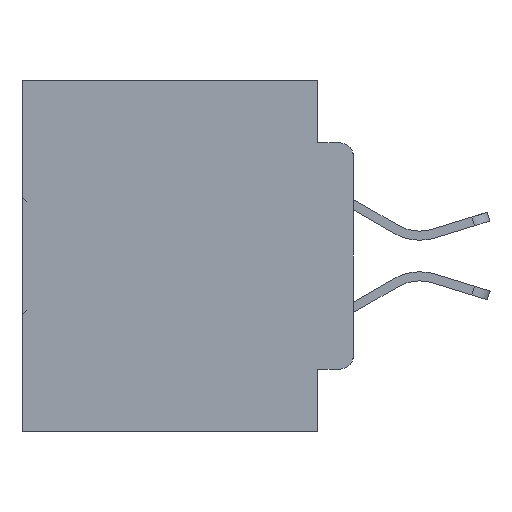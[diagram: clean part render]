
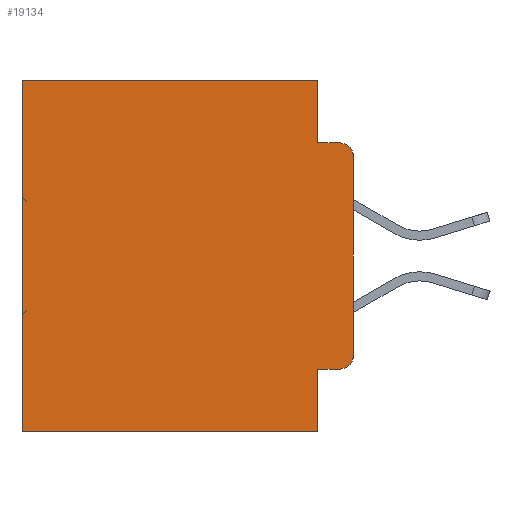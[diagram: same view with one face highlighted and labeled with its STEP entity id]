
A CAD part, left-side view. The second image highlights one B-rep face of the part: STEP entity #19134.
In plain terms, the highlighted planar face has unit normal (-1, 0, 0).
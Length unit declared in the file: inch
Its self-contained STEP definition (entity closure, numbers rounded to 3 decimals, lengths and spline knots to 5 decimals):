
#484 = EDGE_CURVE ( 'NONE', #14846, #5418, #13066, .T. ) ;
#503 = CIRCLE ( 'NONE', #20669, 0.02 ) ;
#848 = PLANE ( 'NONE',  #13218 ) ;
#1187 = LINE ( 'NONE', #32046, #17365 ) ;
#1809 = LINE ( 'NONE', #28675, #14459 ) ;
#2799 = CARTESIAN_POINT ( 'NONE',  ( 0.298, 0.051, 0. ) ) ;
#3646 = VECTOR ( 'NONE', #20056, 39.37008 ) ;
#3702 = VERTEX_POINT ( 'NONE', #13424 ) ;
#3915 = CARTESIAN_POINT ( 'NONE',  ( 0.298, 0., 0. ) ) ;
#3969 = DIRECTION ( 'NONE',  ( 0., -1., 0. ) ) ;
#4075 = EDGE_CURVE ( 'NONE', #13314, #26047, #28355, .T. ) ;
#4445 = ORIENTED_EDGE ( 'NONE', *, *, #15687, .F. ) ;
#4555 = CARTESIAN_POINT ( 'NONE',  ( 0.298, 0.051, -0.5 ) ) ;
#5418 = VERTEX_POINT ( 'NONE', #7967 ) ;
#6611 = VECTOR ( 'NONE', #29232, 39.37008 ) ;
#6970 = EDGE_CURVE ( 'NONE', #30090, #22566, #26677, .T. ) ;
#7066 = DIRECTION ( 'NONE',  ( -1., 0., 0. ) ) ;
#7967 = CARTESIAN_POINT ( 'NONE',  ( 0.298, 0.02, -0.0885 ) ) ;
#8965 = VECTOR ( 'NONE', #35648, 39.37008 ) ;
#8967 = CIRCLE ( 'NONE', #18180, 0.02 ) ;
#9166 = DIRECTION ( 'NONE',  ( 0., 0., -1. ) ) ;
#10667 = LINE ( 'NONE', #12830, #6611 ) ;
#11584 = ORIENTED_EDGE ( 'NONE', *, *, #17065, .F. ) ;
#12199 = DIRECTION ( 'NONE',  ( 0., 0., -1. ) ) ;
#12467 = DIRECTION ( 'NONE',  ( 0., 0., -1. ) ) ;
#12616 = CARTESIAN_POINT ( 'NONE',  ( 0.298, 0., 0. ) ) ;
#12733 = ORIENTED_EDGE ( 'NONE', *, *, #28550, .F. ) ;
#12830 = CARTESIAN_POINT ( 'NONE',  ( 0.298, 0., -0.5 ) ) ;
#13066 = LINE ( 'NONE', #34368, #33563 ) ;
#13218 = AXIS2_PLACEMENT_3D ( 'NONE', #3915, #17276, #9166 ) ;
#13314 = VERTEX_POINT ( 'NONE', #18774 ) ;
#13424 = CARTESIAN_POINT ( 'NONE',  ( 0.298, 0., -0.1085 ) ) ;
#14459 = VECTOR ( 'NONE', #3969, 39.37008 ) ;
#14616 = ORIENTED_EDGE ( 'NONE', *, *, #22593, .T. ) ;
#14752 = FACE_OUTER_BOUND ( 'NONE', #29911, .T. ) ;
#14810 = DIRECTION ( 'NONE',  ( -1., 0., 0. ) ) ;
#14846 = VERTEX_POINT ( 'NONE', #15493 ) ;
#14872 = ORIENTED_EDGE ( 'NONE', *, *, #30583, .T. ) ;
#14900 = CARTESIAN_POINT ( 'NONE',  ( 0.298, 0.473, 0. ) ) ;
#15001 = CARTESIAN_POINT ( 'NONE',  ( 0.298, 0.02, -0.4115 ) ) ;
#15191 = CARTESIAN_POINT ( 'NONE',  ( 0.298, 0.02, -0.1085 ) ) ;
#15493 = CARTESIAN_POINT ( 'NONE',  ( 0.298, 0.051, -0.0885 ) ) ;
#15687 = EDGE_CURVE ( 'NONE', #3702, #35352, #29051, .T. ) ;
#16930 = VERTEX_POINT ( 'NONE', #15001 ) ;
#17065 = EDGE_CURVE ( 'NONE', #26047, #28212, #10667, .T. ) ;
#17276 = DIRECTION ( 'NONE',  ( 1., 0., 0. ) ) ;
#17365 = VECTOR ( 'NONE', #12199, 39.37008 ) ;
#17719 = DIRECTION ( 'NONE',  ( 0., 0., -1. ) ) ;
#18111 = ORIENTED_EDGE ( 'NONE', *, *, #26360, .T. ) ;
#18180 = AXIS2_PLACEMENT_3D ( 'NONE', #28861, #14810, #12467 ) ;
#18306 = VECTOR ( 'NONE', #23601, 39.37008 ) ;
#18650 = DIRECTION ( 'NONE',  ( 0., -1., 0. ) ) ;
#18774 = CARTESIAN_POINT ( 'NONE',  ( 0.298, 0.051, -0.4115 ) ) ;
#19134 = ADVANCED_FACE ( 'NONE', ( #14752 ), #848, .F. ) ;
#19206 = CARTESIAN_POINT ( 'NONE',  ( 0.298, 0., -0.3915 ) ) ;
#20056 = DIRECTION ( 'NONE',  ( 0., 0., -1. ) ) ;
#20244 = DIRECTION ( 'NONE',  ( 0., 0., -1. ) ) ;
#20332 = EDGE_CURVE ( 'NONE', #13314, #16930, #1809, .T. ) ;
#20430 = ORIENTED_EDGE ( 'NONE', *, *, #20332, .T. ) ;
#20669 = AXIS2_PLACEMENT_3D ( 'NONE', #15191, #7066, #20244 ) ;
#21206 = LINE ( 'NONE', #2799, #8965 ) ;
#22397 = VECTOR ( 'NONE', #17719, 39.37008 ) ;
#22566 = VERTEX_POINT ( 'NONE', #14900 ) ;
#22593 = EDGE_CURVE ( 'NONE', #22566, #28212, #1187, .T. ) ;
#22850 = ORIENTED_EDGE ( 'NONE', *, *, #484, .F. ) ;
#23601 = DIRECTION ( 'NONE',  ( 0., 1., 0. ) ) ;
#24132 = CARTESIAN_POINT ( 'NONE',  ( 0.298, 0.473, -0.5 ) ) ;
#25935 = ORIENTED_EDGE ( 'NONE', *, *, #6970, .T. ) ;
#25999 = CARTESIAN_POINT ( 'NONE',  ( 0.298, 0., 0. ) ) ;
#26047 = VERTEX_POINT ( 'NONE', #4555 ) ;
#26360 = EDGE_CURVE ( 'NONE', #16930, #35352, #8967, .T. ) ;
#26677 = LINE ( 'NONE', #12616, #18306 ) ;
#28212 = VERTEX_POINT ( 'NONE', #24132 ) ;
#28355 = LINE ( 'NONE', #28540, #22397 ) ;
#28540 = CARTESIAN_POINT ( 'NONE',  ( 0.298, 0.051, 0. ) ) ;
#28550 = EDGE_CURVE ( 'NONE', #30090, #14846, #21206, .T. ) ;
#28675 = CARTESIAN_POINT ( 'NONE',  ( 0.298, 0.051, -0.4115 ) ) ;
#28861 = CARTESIAN_POINT ( 'NONE',  ( 0.298, 0.02, -0.3915 ) ) ;
#29051 = LINE ( 'NONE', #25999, #3646 ) ;
#29232 = DIRECTION ( 'NONE',  ( 0., 1., 0. ) ) ;
#29911 = EDGE_LOOP ( 'NONE', ( #4445, #14872, #22850, #12733, #25935, #14616, #11584, #31606, #20430, #18111 ) ) ;
#30090 = VERTEX_POINT ( 'NONE', #34905 ) ;
#30583 = EDGE_CURVE ( 'NONE', #3702, #5418, #503, .T. ) ;
#31606 = ORIENTED_EDGE ( 'NONE', *, *, #4075, .F. ) ;
#32046 = CARTESIAN_POINT ( 'NONE',  ( 0.298, 0.473, 0. ) ) ;
#33563 = VECTOR ( 'NONE', #18650, 39.37008 ) ;
#34368 = CARTESIAN_POINT ( 'NONE',  ( 0.298, 0.051, -0.0885 ) ) ;
#34905 = CARTESIAN_POINT ( 'NONE',  ( 0.298, 0.051, 0. ) ) ;
#35352 = VERTEX_POINT ( 'NONE', #19206 ) ;
#35648 = DIRECTION ( 'NONE',  ( 0., 0., -1. ) ) ;
